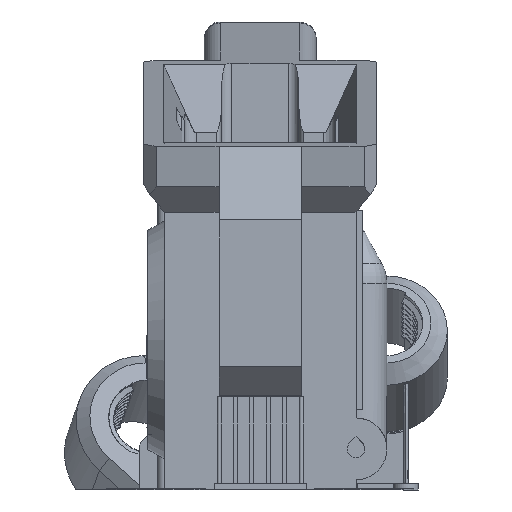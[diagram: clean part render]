
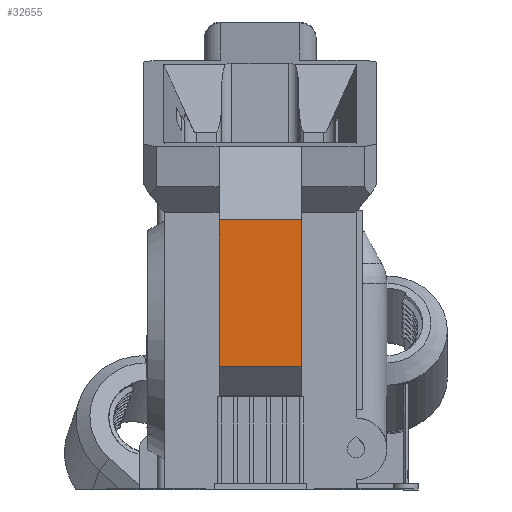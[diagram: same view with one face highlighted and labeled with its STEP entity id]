
A CAD part, left-side view. The second image highlights one B-rep face of the part: STEP entity #32655.
In plain terms, the highlighted planar face has unit normal (-1, 0, 0).
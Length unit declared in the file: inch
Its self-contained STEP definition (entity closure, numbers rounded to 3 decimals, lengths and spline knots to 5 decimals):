
#2779 = DIRECTION ( 'NONE',  ( 0., 1., 0. ) ) ;
#7418 = DIRECTION ( 'NONE',  ( 0., 0., 1. ) ) ;
#19335 = EDGE_CURVE ( 'NONE', #64237, #85083, #109066, .T. ) ;
#32655 = ADVANCED_FACE ( 'NONE', ( #73040 ), #179134, .T. ) ;
#39834 = CARTESIAN_POINT ( 'NONE',  ( -4.237, 0.6526, 1.57821 ) ) ;
#40335 = CARTESIAN_POINT ( 'NONE',  ( -4.237, 0.6526, 2.47116 ) ) ;
#44046 = EDGE_CURVE ( 'NONE', #145362, #89227, #163177, .T. ) ;
#49623 = DIRECTION ( 'NONE',  ( 0., 0., 1. ) ) ;
#51706 = CARTESIAN_POINT ( 'NONE',  ( -4.237, 1.1526, 2.47116 ) ) ;
#53288 = ORIENTED_EDGE ( 'NONE', *, *, #165528, .F. ) ;
#64237 = VERTEX_POINT ( 'NONE', #40335 ) ;
#64539 = CARTESIAN_POINT ( 'NONE',  ( -4.237, 1.1526, 1.52821 ) ) ;
#73040 = FACE_OUTER_BOUND ( 'NONE', #105663, .T. ) ;
#85083 = VERTEX_POINT ( 'NONE', #39834 ) ;
#89227 = VERTEX_POINT ( 'NONE', #51706 ) ;
#93006 = LINE ( 'NONE', #138382, #113186 ) ;
#105663 = EDGE_LOOP ( 'NONE', ( #53288, #184595, #176657, #124088 ) ) ;
#108658 = CARTESIAN_POINT ( 'NONE',  ( -4.237, 2.4558, 1.52821 ) ) ;
#109066 = LINE ( 'NONE', #165357, #127047 ) ;
#111161 = DIRECTION ( 'NONE',  ( 0., 0., -1. ) ) ;
#113186 = VECTOR ( 'NONE', #152225, 39.37008 ) ;
#116914 = AXIS2_PLACEMENT_3D ( 'NONE', #108658, #135709, #49623 ) ;
#117577 = LINE ( 'NONE', #132787, #160759 ) ;
#124088 = ORIENTED_EDGE ( 'NONE', *, *, #44046, .F. ) ;
#127047 = VECTOR ( 'NONE', #111161, 39.37008 ) ;
#129361 = VECTOR ( 'NONE', #7418, 39.37008 ) ;
#132787 = CARTESIAN_POINT ( 'NONE',  ( -4.237, 2.4558, 1.57821 ) ) ;
#135709 = DIRECTION ( 'NONE',  ( -1., 0., 0. ) ) ;
#138382 = CARTESIAN_POINT ( 'NONE',  ( -4.237, 2.4558, 2.47116 ) ) ;
#144566 = EDGE_CURVE ( 'NONE', #89227, #64237, #93006, .T. ) ;
#145362 = VERTEX_POINT ( 'NONE', #164057 ) ;
#152225 = DIRECTION ( 'NONE',  ( 0., -1., 0. ) ) ;
#160759 = VECTOR ( 'NONE', #2779, 39.37008 ) ;
#163177 = LINE ( 'NONE', #64539, #129361 ) ;
#164057 = CARTESIAN_POINT ( 'NONE',  ( -4.237, 1.1526, 1.57821 ) ) ;
#165357 = CARTESIAN_POINT ( 'NONE',  ( -4.237, 0.6526, 1.52821 ) ) ;
#165528 = EDGE_CURVE ( 'NONE', #85083, #145362, #117577, .T. ) ;
#176657 = ORIENTED_EDGE ( 'NONE', *, *, #144566, .F. ) ;
#179134 = PLANE ( 'NONE',  #116914 ) ;
#184595 = ORIENTED_EDGE ( 'NONE', *, *, #19335, .F. ) ;
